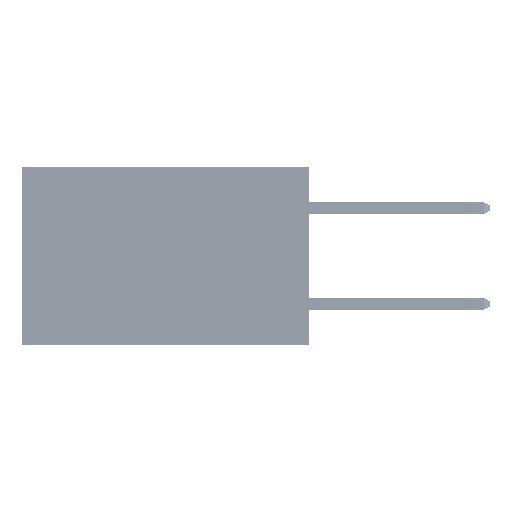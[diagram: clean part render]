
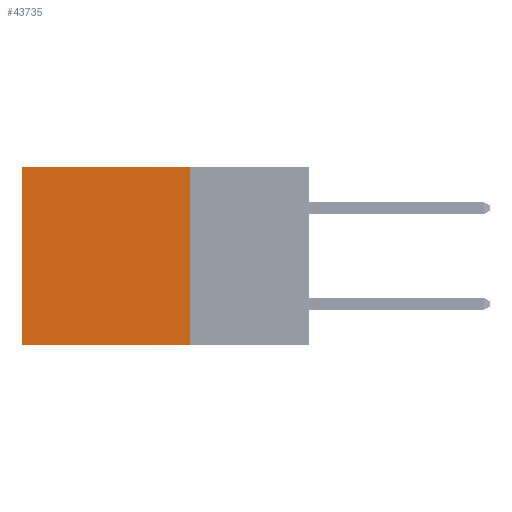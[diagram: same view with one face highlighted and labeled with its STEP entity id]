
A CAD part, left-side view. The second image highlights one B-rep face of the part: STEP entity #43735.
In plain terms, the highlighted planar face has unit normal (-1, 0, 0).
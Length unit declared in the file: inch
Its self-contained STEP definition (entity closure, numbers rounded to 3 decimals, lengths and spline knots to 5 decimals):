
#749 = VERTEX_POINT ( 'NONE', #20574 ) ;
#1676 = ORIENTED_EDGE ( 'NONE', *, *, #29054, .T. ) ;
#2966 = CARTESIAN_POINT ( 'NONE',  ( 0.2875, 0.6, 0. ) ) ;
#3980 = VECTOR ( 'NONE', #43594, 39.37008 ) ;
#6609 = LINE ( 'NONE', #19694, #46816 ) ;
#7296 = DIRECTION ( 'NONE',  ( 0., 0., -1. ) ) ;
#8457 = ORIENTED_EDGE ( 'NONE', *, *, #38843, .F. ) ;
#8750 = EDGE_CURVE ( 'NONE', #749, #28153, #23235, .T. ) ;
#15199 = DIRECTION ( 'NONE',  ( 0., 0., -1. ) ) ;
#18703 = CARTESIAN_POINT ( 'NONE',  ( 0.2875, 0.25, 0. ) ) ;
#19536 = DIRECTION ( 'NONE',  ( 1., 0., 0. ) ) ;
#19694 = CARTESIAN_POINT ( 'NONE',  ( 0.2875, 0.25, 0. ) ) ;
#19869 = DIRECTION ( 'NONE',  ( 0., 1., 0. ) ) ;
#20574 = CARTESIAN_POINT ( 'NONE',  ( 0.2875, 0.6, 0. ) ) ;
#21283 = DIRECTION ( 'NONE',  ( 0., 0., -1. ) ) ;
#22487 = EDGE_CURVE ( 'NONE', #34986, #28153, #23803, .T. ) ;
#22691 = CARTESIAN_POINT ( 'NONE',  ( 0.2875, 0.6, -0.37 ) ) ;
#23219 = PLANE ( 'NONE',  #42118 ) ;
#23235 = LINE ( 'NONE', #2966, #30040 ) ;
#23803 = LINE ( 'NONE', #35012, #3980 ) ;
#24866 = FACE_OUTER_BOUND ( 'NONE', #48798, .T. ) ;
#25315 = LINE ( 'NONE', #29262, #47578 ) ;
#27944 = CARTESIAN_POINT ( 'NONE',  ( 0.2875, 0.25, -0.37 ) ) ;
#28153 = VERTEX_POINT ( 'NONE', #22691 ) ;
#29054 = EDGE_CURVE ( 'NONE', #46295, #749, #6609, .T. ) ;
#29262 = CARTESIAN_POINT ( 'NONE',  ( 0.2875, 0.25, 0. ) ) ;
#30040 = VECTOR ( 'NONE', #15199, 39.37008 ) ;
#30992 = ORIENTED_EDGE ( 'NONE', *, *, #8750, .T. ) ;
#34986 = VERTEX_POINT ( 'NONE', #27944 ) ;
#35012 = CARTESIAN_POINT ( 'NONE',  ( 0.2875, 0.25, -0.37 ) ) ;
#38843 = EDGE_CURVE ( 'NONE', #46295, #34986, #25315, .T. ) ;
#42118 = AXIS2_PLACEMENT_3D ( 'NONE', #47067, #19536, #7296 ) ;
#43594 = DIRECTION ( 'NONE',  ( 0., 1., 0. ) ) ;
#43696 = ORIENTED_EDGE ( 'NONE', *, *, #22487, .F. ) ;
#43735 = ADVANCED_FACE ( 'NONE', ( #24866 ), #23219, .F. ) ;
#46295 = VERTEX_POINT ( 'NONE', #18703 ) ;
#46816 = VECTOR ( 'NONE', #19869, 39.37008 ) ;
#47067 = CARTESIAN_POINT ( 'NONE',  ( 0.2875, 0.25, 0. ) ) ;
#47578 = VECTOR ( 'NONE', #21283, 39.37008 ) ;
#48798 = EDGE_LOOP ( 'NONE', ( #30992, #43696, #8457, #1676 ) ) ;
